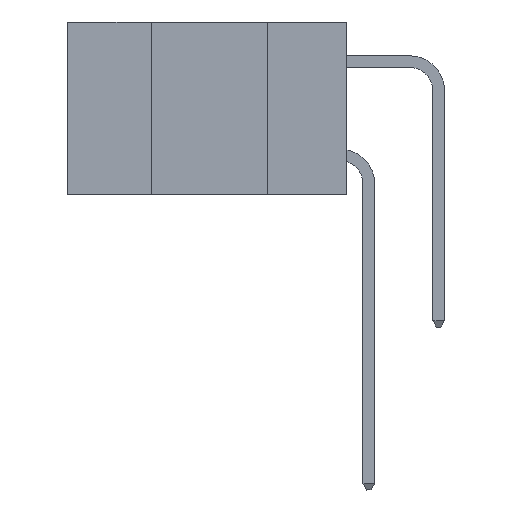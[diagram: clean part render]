
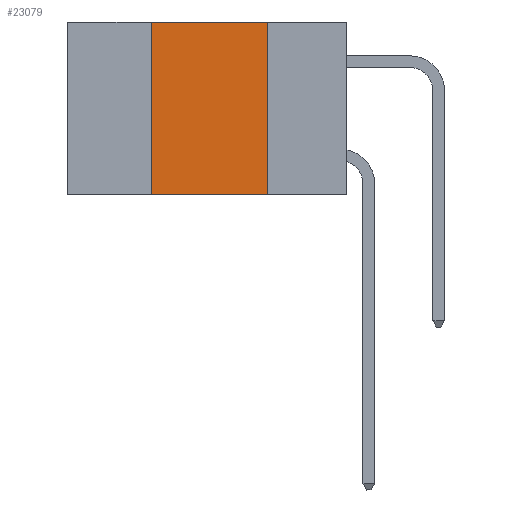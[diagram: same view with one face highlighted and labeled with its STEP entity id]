
A CAD part, left-side view. The second image highlights one B-rep face of the part: STEP entity #23079.
In plain terms, the highlighted planar face has unit normal (-1, 0, 0).
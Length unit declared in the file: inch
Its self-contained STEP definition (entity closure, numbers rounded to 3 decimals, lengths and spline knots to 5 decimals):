
#4742 = EDGE_CURVE ( 'NONE', #7596, #26621, #45053, .T. ) ;
#6101 = CARTESIAN_POINT ( 'NONE',  ( 0., 0.17, 0. ) ) ;
#6541 = ORIENTED_EDGE ( 'NONE', *, *, #38515, .T. ) ;
#6724 = DIRECTION ( 'NONE',  ( 0., -1., 0. ) ) ;
#6914 = DIRECTION ( 'NONE',  ( 1., 0., 0. ) ) ;
#7545 = VECTOR ( 'NONE', #43035, 39.37008 ) ;
#7596 = VERTEX_POINT ( 'NONE', #18167 ) ;
#9181 = ORIENTED_EDGE ( 'NONE', *, *, #39373, .F. ) ;
#9615 = VECTOR ( 'NONE', #40058, 39.37008 ) ;
#13264 = CARTESIAN_POINT ( 'NONE',  ( 0., 0.42, -0.37 ) ) ;
#13738 = CARTESIAN_POINT ( 'NONE',  ( 0., 0.6, 0. ) ) ;
#13828 = DIRECTION ( 'NONE',  ( 0., -1., 0. ) ) ;
#14924 = ORIENTED_EDGE ( 'NONE', *, *, #20936, .F. ) ;
#18167 = CARTESIAN_POINT ( 'NONE',  ( 0., 0.42, 0. ) ) ;
#20936 = EDGE_CURVE ( 'NONE', #45254, #7596, #31958, .T. ) ;
#21035 = CARTESIAN_POINT ( 'NONE',  ( 0., 0.6, -0.37 ) ) ;
#23079 = ADVANCED_FACE ( 'NONE', ( #42978 ), #42582, .F. ) ;
#26621 = VERTEX_POINT ( 'NONE', #6101 ) ;
#27092 = VECTOR ( 'NONE', #6724, 39.37008 ) ;
#28441 = CARTESIAN_POINT ( 'NONE',  ( 0., 0.17, 0. ) ) ;
#28771 = LINE ( 'NONE', #28441, #7545 ) ;
#31580 = CARTESIAN_POINT ( 'NONE',  ( 0., 0.6, 0. ) ) ;
#31958 = LINE ( 'NONE', #32944, #9615 ) ;
#32218 = VECTOR ( 'NONE', #13828, 39.37008 ) ;
#32944 = CARTESIAN_POINT ( 'NONE',  ( 0., 0.42, 0. ) ) ;
#36954 = VERTEX_POINT ( 'NONE', #42698 ) ;
#37181 = ORIENTED_EDGE ( 'NONE', *, *, #4742, .F. ) ;
#37263 = AXIS2_PLACEMENT_3D ( 'NONE', #31580, #6914, #42284 ) ;
#38515 = EDGE_CURVE ( 'NONE', #45254, #36954, #43467, .T. ) ;
#39373 = EDGE_CURVE ( 'NONE', #26621, #36954, #28771, .T. ) ;
#39417 = EDGE_LOOP ( 'NONE', ( #9181, #37181, #14924, #6541 ) ) ;
#40058 = DIRECTION ( 'NONE',  ( 0., 0., 1. ) ) ;
#42284 = DIRECTION ( 'NONE',  ( 0., 0., -1. ) ) ;
#42582 = PLANE ( 'NONE',  #37263 ) ;
#42698 = CARTESIAN_POINT ( 'NONE',  ( 0., 0.17, -0.37 ) ) ;
#42978 = FACE_OUTER_BOUND ( 'NONE', #39417, .T. ) ;
#43035 = DIRECTION ( 'NONE',  ( 0., 0., -1. ) ) ;
#43467 = LINE ( 'NONE', #21035, #32218 ) ;
#45053 = LINE ( 'NONE', #13738, #27092 ) ;
#45254 = VERTEX_POINT ( 'NONE', #13264 ) ;
